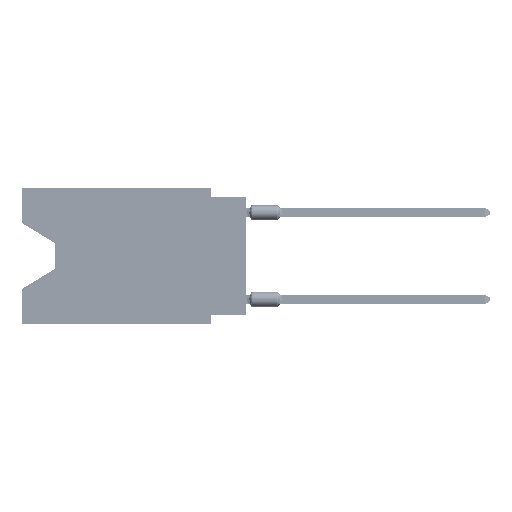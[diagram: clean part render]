
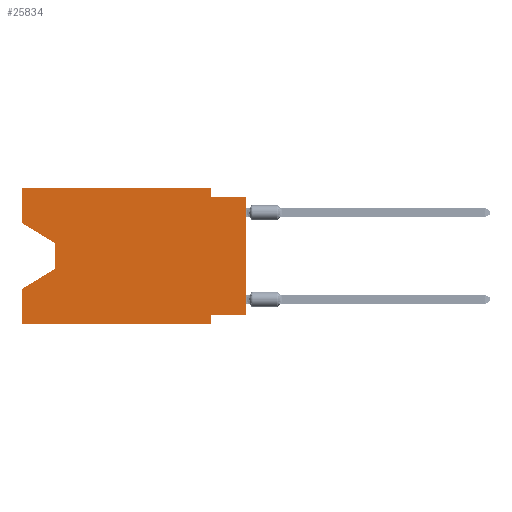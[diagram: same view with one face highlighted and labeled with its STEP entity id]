
A CAD part, left-side view. The second image highlights one B-rep face of the part: STEP entity #25834.
In plain terms, the highlighted planar face has unit normal (-1, 0, 0).
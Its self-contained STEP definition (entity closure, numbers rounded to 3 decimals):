
#398 = VECTOR ( 'NONE', #21037, 1000. ) ;
#767 = LINE ( 'NONE', #54602, #43017 ) ;
#2437 = LINE ( 'NONE', #10796, #22922 ) ;
#2925 = DIRECTION ( 'NONE',  ( 1., 0., 0. ) ) ;
#3117 = CARTESIAN_POINT ( 'NONE',  ( 0., 16.383, 0. ) ) ;
#5619 = CARTESIAN_POINT ( 'NONE',  ( 0., 16.383, 0. ) ) ;
#6483 = ORIENTED_EDGE ( 'NONE', *, *, #25696, .F. ) ;
#7045 = VERTEX_POINT ( 'NONE', #32102 ) ;
#7286 = EDGE_CURVE ( 'NONE', #12293, #74071, #55890, .T. ) ;
#7838 = VECTOR ( 'NONE', #67938, 1000. ) ;
#9663 = CARTESIAN_POINT ( 'NONE',  ( 0., 0., 0. ) ) ;
#9745 = LINE ( 'NONE', #3117, #21941 ) ;
#10796 = CARTESIAN_POINT ( 'NONE',  ( 0., 2.54, -9.906 ) ) ;
#10934 = CARTESIAN_POINT ( 'NONE',  ( 0., 0., -0.635 ) ) ;
#11184 = DIRECTION ( 'NONE',  ( 0., 0., 1. ) ) ;
#11606 = DIRECTION ( 'NONE',  ( 0., -1., 0. ) ) ;
#11895 = EDGE_CURVE ( 'NONE', #64544, #74071, #85988, .T. ) ;
#12293 = VERTEX_POINT ( 'NONE', #23213 ) ;
#13373 = VECTOR ( 'NONE', #66965, 1000. ) ;
#13908 = VECTOR ( 'NONE', #25532, 1000. ) ;
#14088 = LINE ( 'NONE', #67509, #7838 ) ;
#14604 = EDGE_CURVE ( 'NONE', #61924, #45281, #42765, .T. ) ;
#15317 = CARTESIAN_POINT ( 'NONE',  ( 0., 2.54, -0.635 ) ) ;
#15672 = CARTESIAN_POINT ( 'NONE',  ( 0., 16.383, -2.546 ) ) ;
#19041 = VERTEX_POINT ( 'NONE', #50154 ) ;
#19452 = ORIENTED_EDGE ( 'NONE', *, *, #41584, .F. ) ;
#19613 = VECTOR ( 'NONE', #11184, 1000. ) ;
#20359 = CARTESIAN_POINT ( 'NONE',  ( 0., 2.54, -9.271 ) ) ;
#21037 = DIRECTION ( 'NONE',  ( 0., 0.855, -0.519 ) ) ;
#21055 = DIRECTION ( 'NONE',  ( 0., 0., -1. ) ) ;
#21941 = VECTOR ( 'NONE', #57402, 1000. ) ;
#22922 = VECTOR ( 'NONE', #69962, 1000. ) ;
#23213 = CARTESIAN_POINT ( 'NONE',  ( 0., 13.97, -5.893 ) ) ;
#23656 = PLANE ( 'NONE',  #31742 ) ;
#24986 = ORIENTED_EDGE ( 'NONE', *, *, #84966, .F. ) ;
#25532 = DIRECTION ( 'NONE',  ( 0., 0., -1. ) ) ;
#25696 = EDGE_CURVE ( 'NONE', #74323, #50594, #767, .T. ) ;
#25834 = ADVANCED_FACE ( 'NONE', ( #56331 ), #23656, .F. ) ;
#26939 = CARTESIAN_POINT ( 'NONE',  ( 0., 13.97, -4.013 ) ) ;
#27730 = EDGE_LOOP ( 'NONE', ( #50010, #48854, #44314, #86463, #76248, #24986, #19452, #62919, #38217, #6483, #34167, #79467 ) ) ;
#28696 = CARTESIAN_POINT ( 'NONE',  ( 0., 0., -0.635 ) ) ;
#29345 = DIRECTION ( 'NONE',  ( 0., -0.855, -0.519 ) ) ;
#29835 = DIRECTION ( 'NONE',  ( 0., 0., -1. ) ) ;
#30485 = EDGE_CURVE ( 'NONE', #64544, #19041, #65883, .T. ) ;
#31742 = AXIS2_PLACEMENT_3D ( 'NONE', #57211, #2925, #29835 ) ;
#32102 = CARTESIAN_POINT ( 'NONE',  ( 0., 16.383, 0. ) ) ;
#34167 = ORIENTED_EDGE ( 'NONE', *, *, #41347, .F. ) ;
#35843 = VECTOR ( 'NONE', #29345, 1000. ) ;
#38217 = ORIENTED_EDGE ( 'NONE', *, *, #68702, .F. ) ;
#41347 = EDGE_CURVE ( 'NONE', #7045, #74323, #9745, .T. ) ;
#41584 = EDGE_CURVE ( 'NONE', #61924, #53721, #14088, .T. ) ;
#42695 = CARTESIAN_POINT ( 'NONE',  ( 0., 0., -9.271 ) ) ;
#42765 = LINE ( 'NONE', #9663, #71244 ) ;
#43017 = VECTOR ( 'NONE', #21055, 1000. ) ;
#44314 = ORIENTED_EDGE ( 'NONE', *, *, #7286, .T. ) ;
#45281 = VERTEX_POINT ( 'NONE', #10934 ) ;
#46430 = CARTESIAN_POINT ( 'NONE',  ( 0., 16.383, -9.906 ) ) ;
#48854 = ORIENTED_EDGE ( 'NONE', *, *, #86441, .T. ) ;
#50010 = ORIENTED_EDGE ( 'NONE', *, *, #66130, .T. ) ;
#50154 = CARTESIAN_POINT ( 'NONE',  ( 0., 2.54, -9.906 ) ) ;
#50594 = VERTEX_POINT ( 'NONE', #15317 ) ;
#52032 = CARTESIAN_POINT ( 'NONE',  ( 0., 13.97, -4.013 ) ) ;
#52212 = CARTESIAN_POINT ( 'NONE',  ( 0., 16.383, 0. ) ) ;
#52467 = LINE ( 'NONE', #52032, #13908 ) ;
#53721 = VERTEX_POINT ( 'NONE', #20359 ) ;
#54602 = CARTESIAN_POINT ( 'NONE',  ( 0., 2.54, 0. ) ) ;
#55010 = CARTESIAN_POINT ( 'NONE',  ( 0., 13.97, -5.893 ) ) ;
#55890 = LINE ( 'NONE', #55010, #398 ) ;
#56331 = FACE_OUTER_BOUND ( 'NONE', #27730, .T. ) ;
#56477 = LINE ( 'NONE', #28696, #78417 ) ;
#57211 = CARTESIAN_POINT ( 'NONE',  ( 0., 16.383, 0. ) ) ;
#57402 = DIRECTION ( 'NONE',  ( 0., -1., 0. ) ) ;
#57576 = VECTOR ( 'NONE', #11606, 1000. ) ;
#58303 = EDGE_CURVE ( 'NONE', #68760, #7045, #86664, .T. ) ;
#61924 = VERTEX_POINT ( 'NONE', #42695 ) ;
#62919 = ORIENTED_EDGE ( 'NONE', *, *, #14604, .T. ) ;
#63527 = CARTESIAN_POINT ( 'NONE',  ( 0., 16.383, -2.546 ) ) ;
#64544 = VERTEX_POINT ( 'NONE', #71378 ) ;
#65883 = LINE ( 'NONE', #46430, #57576 ) ;
#66130 = EDGE_CURVE ( 'NONE', #68760, #68602, #76606, .T. ) ;
#66965 = DIRECTION ( 'NONE',  ( 0., 0., 1. ) ) ;
#67509 = CARTESIAN_POINT ( 'NONE',  ( 0., 0., -9.271 ) ) ;
#67752 = CARTESIAN_POINT ( 'NONE',  ( 0., 2.54, 0. ) ) ;
#67938 = DIRECTION ( 'NONE',  ( 0., 1., 0. ) ) ;
#68602 = VERTEX_POINT ( 'NONE', #26939 ) ;
#68702 = EDGE_CURVE ( 'NONE', #50594, #45281, #56477, .T. ) ;
#68760 = VERTEX_POINT ( 'NONE', #63527 ) ;
#69705 = DIRECTION ( 'NONE',  ( 0., 0., 1. ) ) ;
#69962 = DIRECTION ( 'NONE',  ( 0., 0., -1. ) ) ;
#71244 = VECTOR ( 'NONE', #69705, 1000. ) ;
#71378 = CARTESIAN_POINT ( 'NONE',  ( 0., 16.383, -9.906 ) ) ;
#74071 = VERTEX_POINT ( 'NONE', #77161 ) ;
#74323 = VERTEX_POINT ( 'NONE', #67752 ) ;
#76248 = ORIENTED_EDGE ( 'NONE', *, *, #30485, .T. ) ;
#76606 = LINE ( 'NONE', #15672, #35843 ) ;
#77161 = CARTESIAN_POINT ( 'NONE',  ( 0., 16.383, -7.36 ) ) ;
#78417 = VECTOR ( 'NONE', #83434, 1000. ) ;
#79467 = ORIENTED_EDGE ( 'NONE', *, *, #58303, .F. ) ;
#83434 = DIRECTION ( 'NONE',  ( 0., -1., 0. ) ) ;
#84966 = EDGE_CURVE ( 'NONE', #53721, #19041, #2437, .T. ) ;
#85988 = LINE ( 'NONE', #5619, #13373 ) ;
#86441 = EDGE_CURVE ( 'NONE', #68602, #12293, #52467, .T. ) ;
#86463 = ORIENTED_EDGE ( 'NONE', *, *, #11895, .F. ) ;
#86664 = LINE ( 'NONE', #52212, #19613 ) ;
